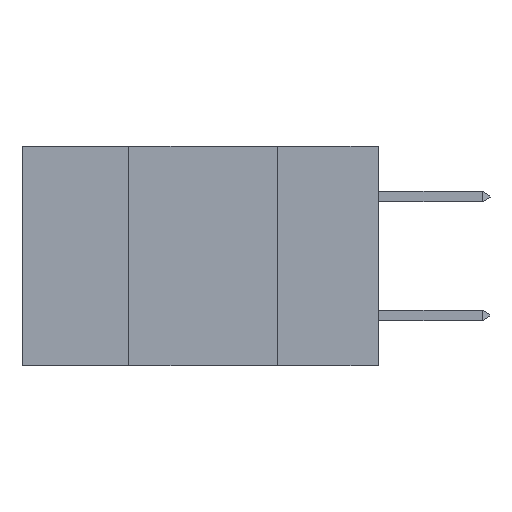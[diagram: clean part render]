
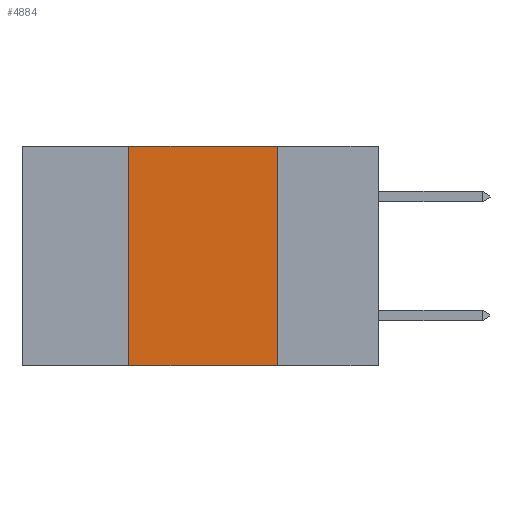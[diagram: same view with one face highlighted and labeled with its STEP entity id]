
A CAD part, left-side view. The second image highlights one B-rep face of the part: STEP entity #4884.
In plain terms, the highlighted planar face has unit normal (-1, 0, 0).
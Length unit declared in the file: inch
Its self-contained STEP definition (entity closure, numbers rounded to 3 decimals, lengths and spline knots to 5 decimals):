
#40 = ORIENTED_EDGE ( 'NONE', *, *, #7429, .T. ) ;
#439 = DIRECTION ( 'NONE',  ( 0., 0., 1. ) ) ;
#1009 = CARTESIAN_POINT ( 'NONE',  ( 0., 0.6, 0. ) ) ;
#1203 = PLANE ( 'NONE',  #1627 ) ;
#1441 = CARTESIAN_POINT ( 'NONE',  ( 0., 0.42, -0.37 ) ) ;
#1627 = AXIS2_PLACEMENT_3D ( 'NONE', #1009, #3389, #2199 ) ;
#2199 = DIRECTION ( 'NONE',  ( 0., 0., -1. ) ) ;
#2380 = CARTESIAN_POINT ( 'NONE',  ( 0., 0.42, 0. ) ) ;
#2617 = LINE ( 'NONE', #8780, #9835 ) ;
#3389 = DIRECTION ( 'NONE',  ( 1., 0., 0. ) ) ;
#3605 = VERTEX_POINT ( 'NONE', #1441 ) ;
#4169 = CARTESIAN_POINT ( 'NONE',  ( 0., 0.6, -0.37 ) ) ;
#4462 = EDGE_LOOP ( 'NONE', ( #7134, #8773, #10928, #40 ) ) ;
#4541 = FACE_OUTER_BOUND ( 'NONE', #4462, .T. ) ;
#4858 = LINE ( 'NONE', #4169, #8916 ) ;
#4884 = ADVANCED_FACE ( 'NONE', ( #4541 ), #1203, .F. ) ;
#5731 = VERTEX_POINT ( 'NONE', #8117 ) ;
#6125 = VECTOR ( 'NONE', #11077, 39.37008 ) ;
#6719 = DIRECTION ( 'NONE',  ( 0., -1., 0. ) ) ;
#7134 = ORIENTED_EDGE ( 'NONE', *, *, #9644, .F. ) ;
#7251 = EDGE_CURVE ( 'NONE', #3605, #14249, #2617, .T. ) ;
#7429 = EDGE_CURVE ( 'NONE', #3605, #5731, #4858, .T. ) ;
#7571 = CARTESIAN_POINT ( 'NONE',  ( 0., 0.17, 0. ) ) ;
#8116 = EDGE_CURVE ( 'NONE', #14249, #11303, #15067, .T. ) ;
#8117 = CARTESIAN_POINT ( 'NONE',  ( 0., 0.17, -0.37 ) ) ;
#8773 = ORIENTED_EDGE ( 'NONE', *, *, #8116, .F. ) ;
#8780 = CARTESIAN_POINT ( 'NONE',  ( 0., 0.42, 0. ) ) ;
#8916 = VECTOR ( 'NONE', #6719, 39.37008 ) ;
#9644 = EDGE_CURVE ( 'NONE', #11303, #5731, #11545, .T. ) ;
#9835 = VECTOR ( 'NONE', #439, 39.37008 ) ;
#10928 = ORIENTED_EDGE ( 'NONE', *, *, #7251, .F. ) ;
#11077 = DIRECTION ( 'NONE',  ( 0., -1., 0. ) ) ;
#11112 = CARTESIAN_POINT ( 'NONE',  ( 0., 0.17, 0. ) ) ;
#11303 = VERTEX_POINT ( 'NONE', #7571 ) ;
#11545 = LINE ( 'NONE', #11112, #13033 ) ;
#12568 = DIRECTION ( 'NONE',  ( 0., 0., -1. ) ) ;
#13033 = VECTOR ( 'NONE', #12568, 39.37008 ) ;
#13319 = CARTESIAN_POINT ( 'NONE',  ( 0., 0.6, 0. ) ) ;
#14249 = VERTEX_POINT ( 'NONE', #2380 ) ;
#15067 = LINE ( 'NONE', #13319, #6125 ) ;
